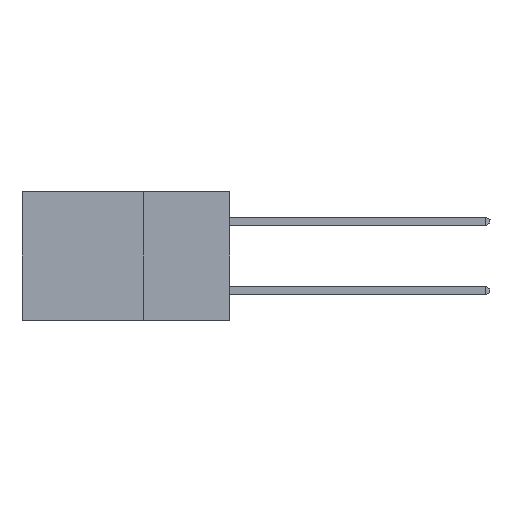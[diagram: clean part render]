
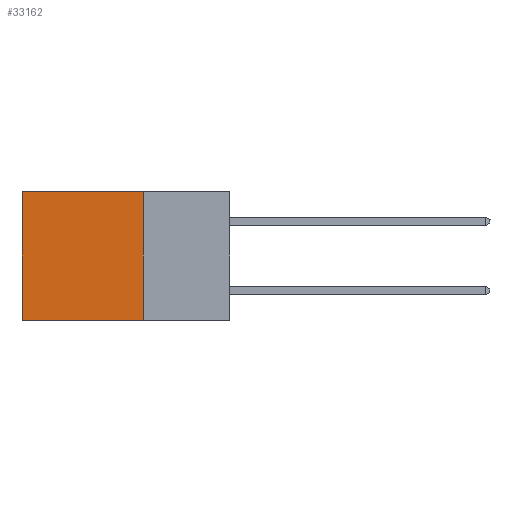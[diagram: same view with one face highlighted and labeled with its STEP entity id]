
A CAD part, left-side view. The second image highlights one B-rep face of the part: STEP entity #33162.
In plain terms, the highlighted planar face has unit normal (-1, 0, 0).
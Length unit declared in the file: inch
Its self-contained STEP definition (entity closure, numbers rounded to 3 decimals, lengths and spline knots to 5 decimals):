
#107 = VECTOR ( 'NONE', #15422, 39.37008 ) ;
#774 = EDGE_CURVE ( 'NONE', #1976, #24823, #10892, .T. ) ;
#1397 = LINE ( 'NONE', #5557, #14406 ) ;
#1976 = VERTEX_POINT ( 'NONE', #27187 ) ;
#5557 = CARTESIAN_POINT ( 'NONE',  ( 0.298, 0.25, -0.37 ) ) ;
#6058 = CARTESIAN_POINT ( 'NONE',  ( 0.298, 0.6, 0. ) ) ;
#7728 = CARTESIAN_POINT ( 'NONE',  ( 0.298, 0.25, -0.37 ) ) ;
#8607 = EDGE_CURVE ( 'NONE', #24823, #18430, #1397, .T. ) ;
#8906 = AXIS2_PLACEMENT_3D ( 'NONE', #29812, #19703, #32554 ) ;
#10694 = DIRECTION ( 'NONE',  ( 0., 1., 0. ) ) ;
#10892 = LINE ( 'NONE', #28511, #33353 ) ;
#14046 = VECTOR ( 'NONE', #22050, 39.37008 ) ;
#14406 = VECTOR ( 'NONE', #10694, 39.37008 ) ;
#15406 = FACE_OUTER_BOUND ( 'NONE', #31454, .T. ) ;
#15422 = DIRECTION ( 'NONE',  ( 0., 1., 0. ) ) ;
#18430 = VERTEX_POINT ( 'NONE', #29594 ) ;
#18757 = CARTESIAN_POINT ( 'NONE',  ( 0.298, 0.6, 0. ) ) ;
#18880 = ORIENTED_EDGE ( 'NONE', *, *, #28396, .T. ) ;
#19162 = ORIENTED_EDGE ( 'NONE', *, *, #774, .F. ) ;
#19703 = DIRECTION ( 'NONE',  ( 1., 0., 0. ) ) ;
#21045 = LINE ( 'NONE', #6058, #14046 ) ;
#22050 = DIRECTION ( 'NONE',  ( 0., 0., -1. ) ) ;
#23414 = LINE ( 'NONE', #28419, #107 ) ;
#24823 = VERTEX_POINT ( 'NONE', #7728 ) ;
#24941 = ORIENTED_EDGE ( 'NONE', *, *, #8607, .F. ) ;
#27187 = CARTESIAN_POINT ( 'NONE',  ( 0.298, 0.25, 0. ) ) ;
#28396 = EDGE_CURVE ( 'NONE', #32266, #18430, #21045, .T. ) ;
#28419 = CARTESIAN_POINT ( 'NONE',  ( 0.298, 0.25, 0. ) ) ;
#28511 = CARTESIAN_POINT ( 'NONE',  ( 0.298, 0.25, 0. ) ) ;
#28962 = DIRECTION ( 'NONE',  ( 0., 0., -1. ) ) ;
#29594 = CARTESIAN_POINT ( 'NONE',  ( 0.298, 0.6, -0.37 ) ) ;
#29604 = EDGE_CURVE ( 'NONE', #1976, #32266, #23414, .T. ) ;
#29812 = CARTESIAN_POINT ( 'NONE',  ( 0.298, 0.25, 0. ) ) ;
#31454 = EDGE_LOOP ( 'NONE', ( #18880, #24941, #19162, #33761 ) ) ;
#32266 = VERTEX_POINT ( 'NONE', #18757 ) ;
#32554 = DIRECTION ( 'NONE',  ( 0., 0., -1. ) ) ;
#32799 = PLANE ( 'NONE',  #8906 ) ;
#33162 = ADVANCED_FACE ( 'NONE', ( #15406 ), #32799, .F. ) ;
#33353 = VECTOR ( 'NONE', #28962, 39.37008 ) ;
#33761 = ORIENTED_EDGE ( 'NONE', *, *, #29604, .T. ) ;
